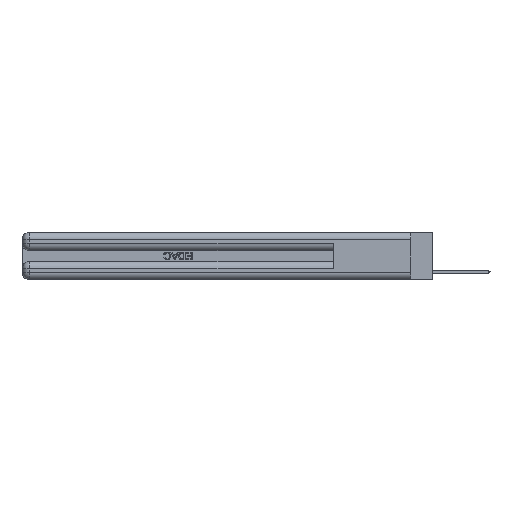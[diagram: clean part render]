
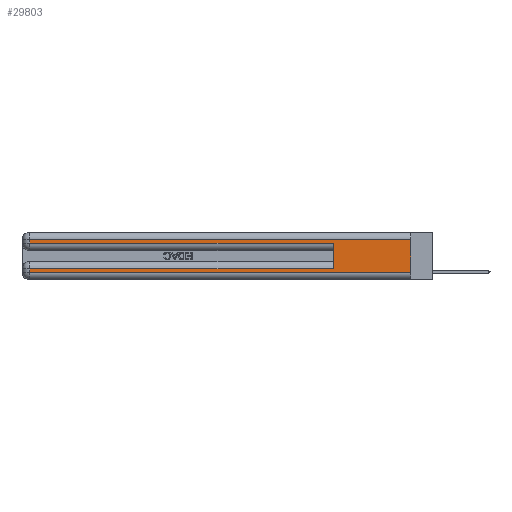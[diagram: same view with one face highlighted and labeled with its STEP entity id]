
A CAD part, left-side view. The second image highlights one B-rep face of the part: STEP entity #29803.
In plain terms, the highlighted planar face has unit normal (-1, 0, 0).
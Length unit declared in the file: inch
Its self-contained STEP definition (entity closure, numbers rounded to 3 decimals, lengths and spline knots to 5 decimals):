
#911 = EDGE_LOOP ( 'NONE', ( #2357, #2120, #6655, #1592, #14802, #2291, #28670, #8698 ) ) ;
#1467 = DIRECTION ( 'NONE',  ( 0., -1., 0. ) ) ;
#1592 = ORIENTED_EDGE ( 'NONE', *, *, #19034, .T. ) ;
#2120 = ORIENTED_EDGE ( 'NONE', *, *, #27445, .T. ) ;
#2291 = ORIENTED_EDGE ( 'NONE', *, *, #31135, .T. ) ;
#2357 = ORIENTED_EDGE ( 'NONE', *, *, #13504, .F. ) ;
#2559 = CARTESIAN_POINT ( 'NONE',  ( 0., 0.6, 0.285 ) ) ;
#2693 = LINE ( 'NONE', #27843, #8342 ) ;
#3788 = VERTEX_POINT ( 'NONE', #5331 ) ;
#3811 = DIRECTION ( 'NONE',  ( 0., 0., 1. ) ) ;
#3917 = AXIS2_PLACEMENT_3D ( 'NONE', #19093, #28830, #14536 ) ;
#4442 = LINE ( 'NONE', #15557, #24865 ) ;
#4842 = VECTOR ( 'NONE', #7155, 39.37008 ) ;
#5137 = LINE ( 'NONE', #10803, #10834 ) ;
#5331 = CARTESIAN_POINT ( 'NONE',  ( 0., 2.94, 0.06 ) ) ;
#6084 = CARTESIAN_POINT ( 'NONE',  ( 0., 0., 0.06 ) ) ;
#6655 = ORIENTED_EDGE ( 'NONE', *, *, #25880, .T. ) ;
#6677 = VERTEX_POINT ( 'NONE', #24337 ) ;
#6881 = FACE_OUTER_BOUND ( 'NONE', #911, .T. ) ;
#7155 = DIRECTION ( 'NONE',  ( 0., -1., 0. ) ) ;
#7472 = VECTOR ( 'NONE', #14478, 39.37008 ) ;
#8179 = CARTESIAN_POINT ( 'NONE',  ( 0., 0., 0.31 ) ) ;
#8342 = VECTOR ( 'NONE', #25633, 39.37008 ) ;
#8698 = ORIENTED_EDGE ( 'NONE', *, *, #12267, .T. ) ;
#8998 = LINE ( 'NONE', #28971, #7472 ) ;
#9026 = CARTESIAN_POINT ( 'NONE',  ( 0., 0., 0.06 ) ) ;
#9262 = EDGE_CURVE ( 'NONE', #29372, #14912, #5137, .T. ) ;
#9968 = CARTESIAN_POINT ( 'NONE',  ( 0., 0., 0.085 ) ) ;
#10225 = LINE ( 'NONE', #9968, #19705 ) ;
#10803 = CARTESIAN_POINT ( 'NONE',  ( 0., 0.6, 0.145 ) ) ;
#10810 = CARTESIAN_POINT ( 'NONE',  ( 0., 2.94, 0.085 ) ) ;
#10834 = VECTOR ( 'NONE', #3811, 39.37008 ) ;
#12267 = EDGE_CURVE ( 'NONE', #3788, #19671, #29259, .T. ) ;
#12499 = VERTEX_POINT ( 'NONE', #8179 ) ;
#13504 = EDGE_CURVE ( 'NONE', #12499, #19671, #2693, .T. ) ;
#14478 = DIRECTION ( 'NONE',  ( 0., 1., 0. ) ) ;
#14536 = DIRECTION ( 'NONE',  ( 0., 0., -1. ) ) ;
#14802 = ORIENTED_EDGE ( 'NONE', *, *, #9262, .F. ) ;
#14912 = VERTEX_POINT ( 'NONE', #2559 ) ;
#15557 = CARTESIAN_POINT ( 'NONE',  ( 0., 2.94, 0.37 ) ) ;
#16256 = LINE ( 'NONE', #16526, #4842 ) ;
#16526 = CARTESIAN_POINT ( 'NONE',  ( 0., 0., 0.285 ) ) ;
#17833 = CARTESIAN_POINT ( 'NONE',  ( 0., 0.6, 0.085 ) ) ;
#18053 = VERTEX_POINT ( 'NONE', #21425 ) ;
#19034 = EDGE_CURVE ( 'NONE', #6677, #14912, #16256, .T. ) ;
#19093 = CARTESIAN_POINT ( 'NONE',  ( 0., 0., 0.37 ) ) ;
#19671 = VERTEX_POINT ( 'NONE', #9026 ) ;
#19705 = VECTOR ( 'NONE', #26615, 39.37008 ) ;
#20615 = DIRECTION ( 'NONE',  ( 0., 0., -1. ) ) ;
#21425 = CARTESIAN_POINT ( 'NONE',  ( 0., 2.94, 0.31 ) ) ;
#21726 = CARTESIAN_POINT ( 'NONE',  ( 0., 2.94, 0.37 ) ) ;
#22798 = VECTOR ( 'NONE', #1467, 39.37008 ) ;
#23813 = DIRECTION ( 'NONE',  ( 0., 0., -1. ) ) ;
#23853 = LINE ( 'NONE', #21726, #29209 ) ;
#23926 = PLANE ( 'NONE',  #3917 ) ;
#24337 = CARTESIAN_POINT ( 'NONE',  ( 0., 2.94, 0.285 ) ) ;
#24865 = VECTOR ( 'NONE', #20615, 39.37008 ) ;
#25633 = DIRECTION ( 'NONE',  ( 0., 0., -1. ) ) ;
#25880 = EDGE_CURVE ( 'NONE', #18053, #6677, #23853, .T. ) ;
#26615 = DIRECTION ( 'NONE',  ( 0., 1., 0. ) ) ;
#27445 = EDGE_CURVE ( 'NONE', #12499, #18053, #8998, .T. ) ;
#27843 = CARTESIAN_POINT ( 'NONE',  ( 0., 0., 0.37 ) ) ;
#28670 = ORIENTED_EDGE ( 'NONE', *, *, #29001, .T. ) ;
#28830 = DIRECTION ( 'NONE',  ( 1., 0., 0. ) ) ;
#28971 = CARTESIAN_POINT ( 'NONE',  ( 0., 0., 0.31 ) ) ;
#29001 = EDGE_CURVE ( 'NONE', #31344, #3788, #4442, .T. ) ;
#29209 = VECTOR ( 'NONE', #23813, 39.37008 ) ;
#29259 = LINE ( 'NONE', #6084, #22798 ) ;
#29372 = VERTEX_POINT ( 'NONE', #17833 ) ;
#29803 = ADVANCED_FACE ( 'NONE', ( #6881 ), #23926, .F. ) ;
#31135 = EDGE_CURVE ( 'NONE', #29372, #31344, #10225, .T. ) ;
#31344 = VERTEX_POINT ( 'NONE', #10810 ) ;
